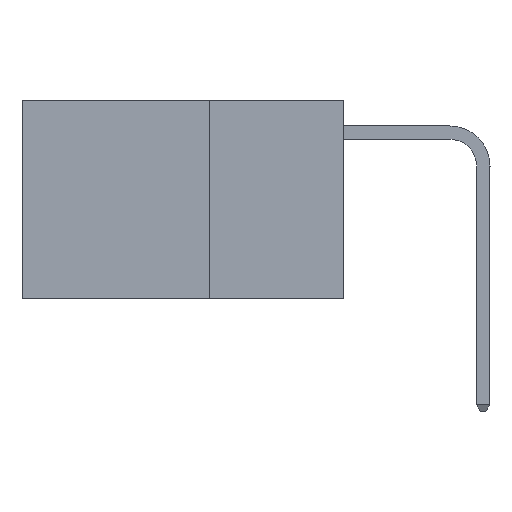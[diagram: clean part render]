
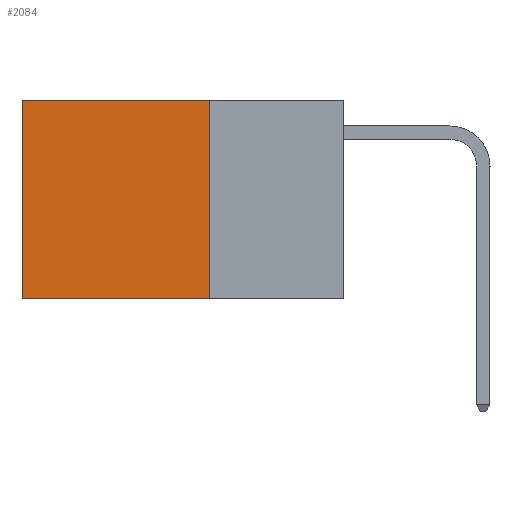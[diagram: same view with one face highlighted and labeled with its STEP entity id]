
A CAD part, left-side view. The second image highlights one B-rep face of the part: STEP entity #2084.
In plain terms, the highlighted planar face has unit normal (-1, 0, 0).
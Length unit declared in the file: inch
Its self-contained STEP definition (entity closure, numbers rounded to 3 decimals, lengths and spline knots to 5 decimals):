
#283 = EDGE_CURVE ( 'NONE', #18563, #7818, #20374, .T. ) ;
#575 = LINE ( 'NONE', #13667, #11750 ) ;
#1100 = DIRECTION ( 'NONE',  ( 0., 1., 0. ) ) ;
#1414 = ORIENTED_EDGE ( 'NONE', *, *, #6369, .F. ) ;
#1691 = CARTESIAN_POINT ( 'NONE',  ( 0.2625, 0.25, -0.37 ) ) ;
#2044 = CARTESIAN_POINT ( 'NONE',  ( 0.2625, 0.6, -0.37 ) ) ;
#2084 = ADVANCED_FACE ( 'NONE', ( #23977 ), #16544, .F. ) ;
#2227 = DIRECTION ( 'NONE',  ( 0., 0., -1. ) ) ;
#2596 = LINE ( 'NONE', #1691, #3940 ) ;
#3679 = EDGE_LOOP ( 'NONE', ( #10040, #23430, #1414, #24775 ) ) ;
#3940 = VECTOR ( 'NONE', #12131, 39.37008 ) ;
#4060 = DIRECTION ( 'NONE',  ( 1., 0., 0. ) ) ;
#4428 = VECTOR ( 'NONE', #13616, 39.37008 ) ;
#6369 = EDGE_CURVE ( 'NONE', #19620, #9232, #18305, .T. ) ;
#6390 = CARTESIAN_POINT ( 'NONE',  ( 0.2625, 0.25, 0. ) ) ;
#7818 = VERTEX_POINT ( 'NONE', #2044 ) ;
#9232 = VERTEX_POINT ( 'NONE', #25004 ) ;
#10040 = ORIENTED_EDGE ( 'NONE', *, *, #283, .T. ) ;
#11750 = VECTOR ( 'NONE', #1100, 39.37008 ) ;
#11959 = EDGE_CURVE ( 'NONE', #9232, #7818, #2596, .T. ) ;
#12131 = DIRECTION ( 'NONE',  ( 0., 1., 0. ) ) ;
#12790 = VECTOR ( 'NONE', #2227, 39.37008 ) ;
#13468 = CARTESIAN_POINT ( 'NONE',  ( 0.2625, 0.6, 0. ) ) ;
#13616 = DIRECTION ( 'NONE',  ( 0., 0., -1. ) ) ;
#13667 = CARTESIAN_POINT ( 'NONE',  ( 0.2625, 0.25, 0. ) ) ;
#16184 = CARTESIAN_POINT ( 'NONE',  ( 0.2625, 0.6, 0. ) ) ;
#16544 = PLANE ( 'NONE',  #23584 ) ;
#18305 = LINE ( 'NONE', #6390, #12790 ) ;
#18511 = CARTESIAN_POINT ( 'NONE',  ( 0.2625, 0.25, 0. ) ) ;
#18563 = VERTEX_POINT ( 'NONE', #16184 ) ;
#18606 = DIRECTION ( 'NONE',  ( 0., 0., -1. ) ) ;
#19620 = VERTEX_POINT ( 'NONE', #25169 ) ;
#19865 = EDGE_CURVE ( 'NONE', #19620, #18563, #575, .T. ) ;
#20374 = LINE ( 'NONE', #13468, #4428 ) ;
#23430 = ORIENTED_EDGE ( 'NONE', *, *, #11959, .F. ) ;
#23584 = AXIS2_PLACEMENT_3D ( 'NONE', #18511, #4060, #18606 ) ;
#23977 = FACE_OUTER_BOUND ( 'NONE', #3679, .T. ) ;
#24775 = ORIENTED_EDGE ( 'NONE', *, *, #19865, .T. ) ;
#25004 = CARTESIAN_POINT ( 'NONE',  ( 0.2625, 0.25, -0.37 ) ) ;
#25169 = CARTESIAN_POINT ( 'NONE',  ( 0.2625, 0.25, 0. ) ) ;
